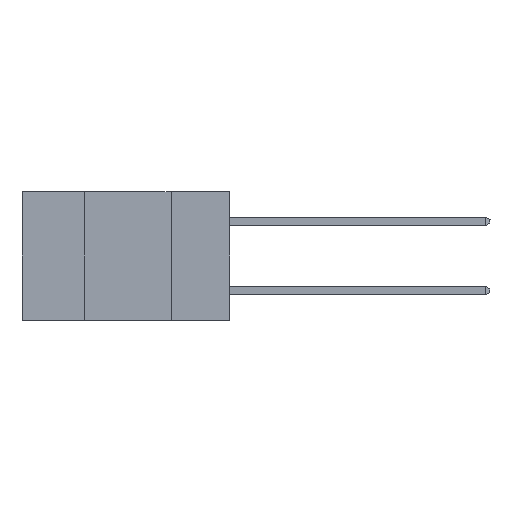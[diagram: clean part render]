
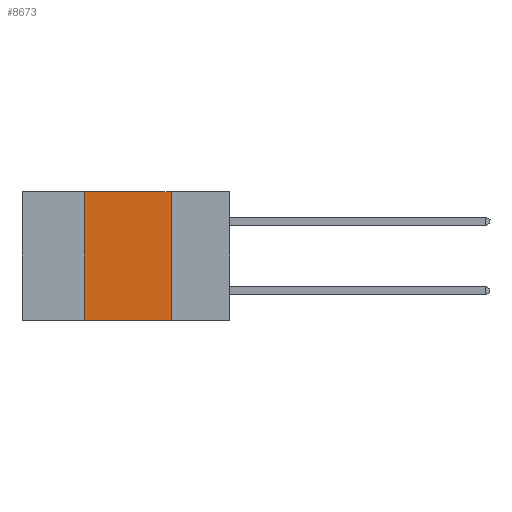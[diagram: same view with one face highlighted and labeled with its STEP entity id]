
A CAD part, left-side view. The second image highlights one B-rep face of the part: STEP entity #8673.
In plain terms, the highlighted planar face has unit normal (-1, 0, 0).
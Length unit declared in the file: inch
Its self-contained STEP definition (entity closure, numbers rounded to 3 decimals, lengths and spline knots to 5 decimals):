
#135 = CARTESIAN_POINT ( 'NONE',  ( 0., 0.42, 0. ) ) ;
#503 = ORIENTED_EDGE ( 'NONE', *, *, #4752, .T. ) ;
#945 = PLANE ( 'NONE',  #12051 ) ;
#1087 = EDGE_CURVE ( 'NONE', #1194, #1547, #1841, .T. ) ;
#1194 = VERTEX_POINT ( 'NONE', #2088 ) ;
#1547 = VERTEX_POINT ( 'NONE', #8369 ) ;
#1841 = LINE ( 'NONE', #9828, #8699 ) ;
#1884 = ORIENTED_EDGE ( 'NONE', *, *, #4844, .F. ) ;
#1971 = DIRECTION ( 'NONE',  ( 1., 0., 0. ) ) ;
#2088 = CARTESIAN_POINT ( 'NONE',  ( 0., 0.17, 0. ) ) ;
#3894 = DIRECTION ( 'NONE',  ( 0., -1., 0. ) ) ;
#4752 = EDGE_CURVE ( 'NONE', #5611, #1547, #7782, .T. ) ;
#4773 = DIRECTION ( 'NONE',  ( 0., 0., -1. ) ) ;
#4844 = EDGE_CURVE ( 'NONE', #6251, #1194, #7843, .T. ) ;
#4878 = EDGE_LOOP ( 'NONE', ( #8613, #1884, #8157, #503 ) ) ;
#4904 = CARTESIAN_POINT ( 'NONE',  ( 0., 0.6, 0. ) ) ;
#5215 = VECTOR ( 'NONE', #6366, 39.37008 ) ;
#5512 = VECTOR ( 'NONE', #3894, 39.37008 ) ;
#5611 = VERTEX_POINT ( 'NONE', #7412 ) ;
#5802 = DIRECTION ( 'NONE',  ( 0., 0., -1. ) ) ;
#6251 = VERTEX_POINT ( 'NONE', #135 ) ;
#6366 = DIRECTION ( 'NONE',  ( 0., 0., 1. ) ) ;
#6911 = FACE_OUTER_BOUND ( 'NONE', #4878, .T. ) ;
#7412 = CARTESIAN_POINT ( 'NONE',  ( 0., 0.42, -0.37 ) ) ;
#7460 = EDGE_CURVE ( 'NONE', #5611, #6251, #11028, .T. ) ;
#7714 = DIRECTION ( 'NONE',  ( 0., -1., 0. ) ) ;
#7782 = LINE ( 'NONE', #8574, #5512 ) ;
#7843 = LINE ( 'NONE', #12758, #11368 ) ;
#8157 = ORIENTED_EDGE ( 'NONE', *, *, #7460, .F. ) ;
#8369 = CARTESIAN_POINT ( 'NONE',  ( 0., 0.17, -0.37 ) ) ;
#8574 = CARTESIAN_POINT ( 'NONE',  ( 0., 0.6, -0.37 ) ) ;
#8613 = ORIENTED_EDGE ( 'NONE', *, *, #1087, .F. ) ;
#8673 = ADVANCED_FACE ( 'NONE', ( #6911 ), #945, .F. ) ;
#8699 = VECTOR ( 'NONE', #5802, 39.37008 ) ;
#9345 = CARTESIAN_POINT ( 'NONE',  ( 0., 0.42, -0.37 ) ) ;
#9828 = CARTESIAN_POINT ( 'NONE',  ( 0., 0.17, -0.37 ) ) ;
#11028 = LINE ( 'NONE', #9345, #5215 ) ;
#11368 = VECTOR ( 'NONE', #7714, 39.37008 ) ;
#12051 = AXIS2_PLACEMENT_3D ( 'NONE', #4904, #1971, #4773 ) ;
#12758 = CARTESIAN_POINT ( 'NONE',  ( 0., 0.6, 0. ) ) ;
